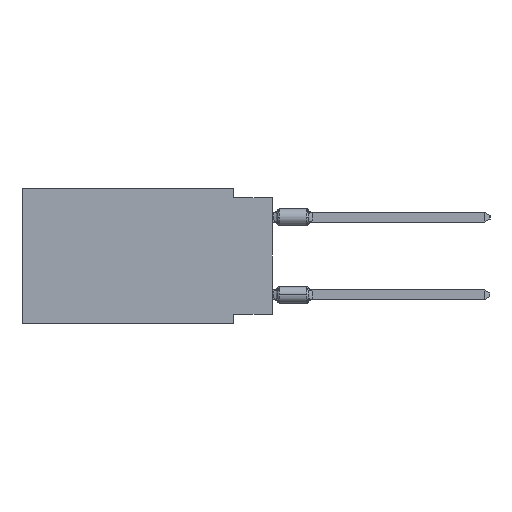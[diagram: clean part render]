
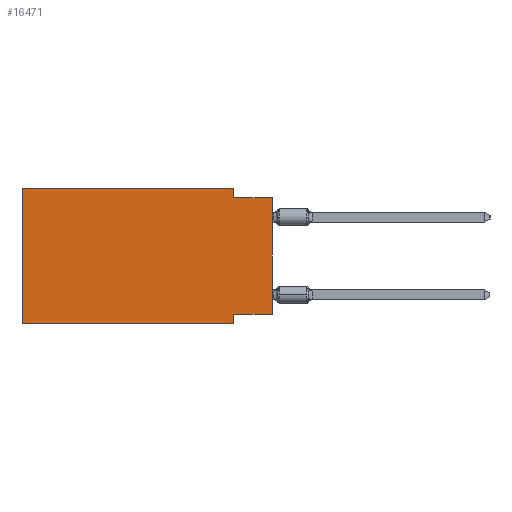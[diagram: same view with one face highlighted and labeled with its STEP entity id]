
A CAD part, left-side view. The second image highlights one B-rep face of the part: STEP entity #16471.
In plain terms, the highlighted planar face has unit normal (-1, 0, 0).
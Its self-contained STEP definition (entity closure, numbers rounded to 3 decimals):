
#372 = CARTESIAN_POINT ( 'NONE',  ( 0., 16.383, -8.89 ) ) ;
#1165 = EDGE_CURVE ( 'NONE', #10396, #30719, #8678, .T. ) ;
#1290 = CARTESIAN_POINT ( 'NONE',  ( 0., 0., -0.635 ) ) ;
#1413 = PLANE ( 'NONE',  #20161 ) ;
#1625 = CARTESIAN_POINT ( 'NONE',  ( 0., 16.383, 0. ) ) ;
#1628 = LINE ( 'NONE', #26863, #5514 ) ;
#1643 = VECTOR ( 'NONE', #14332, 1000. ) ;
#2059 = ORIENTED_EDGE ( 'NONE', *, *, #13462, .T. ) ;
#3273 = CARTESIAN_POINT ( 'NONE',  ( 0., 0., -8.255 ) ) ;
#3451 = ORIENTED_EDGE ( 'NONE', *, *, #26539, .F. ) ;
#3682 = CARTESIAN_POINT ( 'NONE',  ( 0., 0., 0. ) ) ;
#3730 = LINE ( 'NONE', #13769, #4769 ) ;
#3741 = FACE_OUTER_BOUND ( 'NONE', #30113, .T. ) ;
#3891 = DIRECTION ( 'NONE',  ( 0., 0., -1. ) ) ;
#4422 = ORIENTED_EDGE ( 'NONE', *, *, #24461, .F. ) ;
#4599 = CARTESIAN_POINT ( 'NONE',  ( 0., 2.54, -8.89 ) ) ;
#4769 = VECTOR ( 'NONE', #23332, 1000. ) ;
#4771 = CARTESIAN_POINT ( 'NONE',  ( 0., 0., -0.635 ) ) ;
#5026 = CARTESIAN_POINT ( 'NONE',  ( 0., 0., -8.255 ) ) ;
#5323 = CARTESIAN_POINT ( 'NONE',  ( 0., 2.54, 0. ) ) ;
#5514 = VECTOR ( 'NONE', #14161, 1000. ) ;
#5726 = VECTOR ( 'NONE', #15565, 1000. ) ;
#6500 = CARTESIAN_POINT ( 'NONE',  ( 0., 2.54, -8.255 ) ) ;
#6583 = VECTOR ( 'NONE', #3891, 1000. ) ;
#6735 = LINE ( 'NONE', #4771, #1643 ) ;
#6755 = EDGE_CURVE ( 'NONE', #30719, #17333, #6735, .T. ) ;
#8678 = LINE ( 'NONE', #21186, #6583 ) ;
#8897 = VERTEX_POINT ( 'NONE', #6500 ) ;
#10324 = CARTESIAN_POINT ( 'NONE',  ( 0., 16.383, -8.89 ) ) ;
#10346 = ORIENTED_EDGE ( 'NONE', *, *, #32320, .T. ) ;
#10396 = VERTEX_POINT ( 'NONE', #5323 ) ;
#10937 = EDGE_CURVE ( 'NONE', #23281, #10396, #1628, .T. ) ;
#12154 = VECTOR ( 'NONE', #24979, 1000. ) ;
#12866 = VERTEX_POINT ( 'NONE', #10324 ) ;
#13462 = EDGE_CURVE ( 'NONE', #31836, #17333, #28400, .T. ) ;
#13769 = CARTESIAN_POINT ( 'NONE',  ( 0., 2.54, -8.89 ) ) ;
#13950 = DIRECTION ( 'NONE',  ( 1., 0., 0. ) ) ;
#14161 = DIRECTION ( 'NONE',  ( 0., -1., 0. ) ) ;
#14332 = DIRECTION ( 'NONE',  ( 0., -1., 0. ) ) ;
#14428 = CARTESIAN_POINT ( 'NONE',  ( 0., 2.54, -0.635 ) ) ;
#15565 = DIRECTION ( 'NONE',  ( 0., -1., 0. ) ) ;
#15653 = ORIENTED_EDGE ( 'NONE', *, *, #1165, .F. ) ;
#16471 = ADVANCED_FACE ( 'NONE', ( #3741 ), #1413, .F. ) ;
#16541 = DIRECTION ( 'NONE',  ( 0., 0., 1. ) ) ;
#17333 = VERTEX_POINT ( 'NONE', #1290 ) ;
#18588 = VERTEX_POINT ( 'NONE', #4599 ) ;
#20161 = AXIS2_PLACEMENT_3D ( 'NONE', #23678, #13950, #29096 ) ;
#20652 = LINE ( 'NONE', #372, #5726 ) ;
#21186 = CARTESIAN_POINT ( 'NONE',  ( 0., 2.54, 0. ) ) ;
#23281 = VERTEX_POINT ( 'NONE', #25974 ) ;
#23332 = DIRECTION ( 'NONE',  ( 0., 0., -1. ) ) ;
#23653 = VECTOR ( 'NONE', #26372, 1000. ) ;
#23678 = CARTESIAN_POINT ( 'NONE',  ( 0., 16.383, 0. ) ) ;
#24219 = LINE ( 'NONE', #1625, #23653 ) ;
#24461 = EDGE_CURVE ( 'NONE', #8897, #18588, #3730, .T. ) ;
#24804 = EDGE_CURVE ( 'NONE', #31836, #8897, #29742, .T. ) ;
#24979 = DIRECTION ( 'NONE',  ( 0., 1., 0. ) ) ;
#25704 = ORIENTED_EDGE ( 'NONE', *, *, #10937, .F. ) ;
#25974 = CARTESIAN_POINT ( 'NONE',  ( 0., 16.383, 0. ) ) ;
#26372 = DIRECTION ( 'NONE',  ( 0., 0., 1. ) ) ;
#26539 = EDGE_CURVE ( 'NONE', #12866, #23281, #24219, .T. ) ;
#26863 = CARTESIAN_POINT ( 'NONE',  ( 0., 16.383, 0. ) ) ;
#27820 = ORIENTED_EDGE ( 'NONE', *, *, #24804, .F. ) ;
#28400 = LINE ( 'NONE', #3682, #28759 ) ;
#28759 = VECTOR ( 'NONE', #16541, 1000. ) ;
#29096 = DIRECTION ( 'NONE',  ( 0., 0., -1. ) ) ;
#29742 = LINE ( 'NONE', #5026, #12154 ) ;
#30113 = EDGE_LOOP ( 'NONE', ( #2059, #31458, #15653, #25704, #3451, #10346, #4422, #27820 ) ) ;
#30719 = VERTEX_POINT ( 'NONE', #14428 ) ;
#31458 = ORIENTED_EDGE ( 'NONE', *, *, #6755, .F. ) ;
#31836 = VERTEX_POINT ( 'NONE', #3273 ) ;
#32320 = EDGE_CURVE ( 'NONE', #12866, #18588, #20652, .T. ) ;
